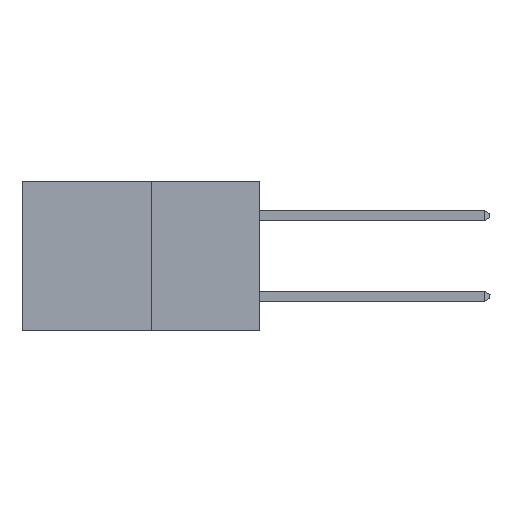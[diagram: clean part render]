
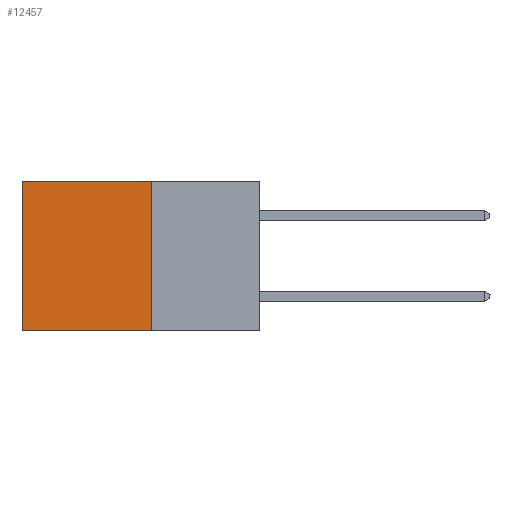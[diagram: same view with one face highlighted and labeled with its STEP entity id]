
A CAD part, left-side view. The second image highlights one B-rep face of the part: STEP entity #12457.
In plain terms, the highlighted planar face has unit normal (-1, 0, 0).
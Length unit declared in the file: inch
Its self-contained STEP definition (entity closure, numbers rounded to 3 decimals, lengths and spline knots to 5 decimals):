
#327 = VERTEX_POINT ( 'NONE', #22577 ) ;
#409 = VERTEX_POINT ( 'NONE', #3282 ) ;
#565 = VERTEX_POINT ( 'NONE', #15094 ) ;
#686 = ORIENTED_EDGE ( 'NONE', *, *, #25477, .T. ) ;
#914 = CARTESIAN_POINT ( 'NONE',  ( 0.277, 0.59, -0.37 ) ) ;
#937 = FACE_OUTER_BOUND ( 'NONE', #2817, .T. ) ;
#1234 = DIRECTION ( 'NONE',  ( 0., 1., 0. ) ) ;
#1362 = LINE ( 'NONE', #26528, #12355 ) ;
#2286 = DIRECTION ( 'NONE',  ( 0., 0., -1. ) ) ;
#2817 = EDGE_LOOP ( 'NONE', ( #7984, #17784, #15500, #686 ) ) ;
#3172 = DIRECTION ( 'NONE',  ( 0., 0., -1. ) ) ;
#3282 = CARTESIAN_POINT ( 'NONE',  ( 0.277, 0.59, 0. ) ) ;
#7818 = CARTESIAN_POINT ( 'NONE',  ( 0.277, 0.27, -0.37 ) ) ;
#7984 = ORIENTED_EDGE ( 'NONE', *, *, #8942, .T. ) ;
#8942 = EDGE_CURVE ( 'NONE', #409, #565, #15230, .T. ) ;
#10881 = VERTEX_POINT ( 'NONE', #18780 ) ;
#11003 = PLANE ( 'NONE',  #18610 ) ;
#12355 = VECTOR ( 'NONE', #22347, 39.37008 ) ;
#12457 = ADVANCED_FACE ( 'NONE', ( #937 ), #11003, .F. ) ;
#15094 = CARTESIAN_POINT ( 'NONE',  ( 0.277, 0.59, -0.37 ) ) ;
#15230 = LINE ( 'NONE', #914, #25888 ) ;
#15355 = DIRECTION ( 'NONE',  ( 1., 0., 0. ) ) ;
#15500 = ORIENTED_EDGE ( 'NONE', *, *, #17547, .F. ) ;
#15741 = VECTOR ( 'NONE', #25037, 39.37008 ) ;
#17052 = EDGE_CURVE ( 'NONE', #10881, #565, #25071, .T. ) ;
#17415 = CARTESIAN_POINT ( 'NONE',  ( 0.277, 0.27, -0.37 ) ) ;
#17547 = EDGE_CURVE ( 'NONE', #327, #10881, #1362, .T. ) ;
#17784 = ORIENTED_EDGE ( 'NONE', *, *, #17052, .F. ) ;
#18610 = AXIS2_PLACEMENT_3D ( 'NONE', #17415, #15355, #2286 ) ;
#18780 = CARTESIAN_POINT ( 'NONE',  ( 0.277, 0.27, -0.37 ) ) ;
#19413 = VECTOR ( 'NONE', #1234, 39.37008 ) ;
#20725 = LINE ( 'NONE', #22914, #15741 ) ;
#22347 = DIRECTION ( 'NONE',  ( 0., 0., -1. ) ) ;
#22577 = CARTESIAN_POINT ( 'NONE',  ( 0.277, 0.27, 0. ) ) ;
#22914 = CARTESIAN_POINT ( 'NONE',  ( 0.277, 0.27, 0. ) ) ;
#25037 = DIRECTION ( 'NONE',  ( 0., 1., 0. ) ) ;
#25071 = LINE ( 'NONE', #7818, #19413 ) ;
#25477 = EDGE_CURVE ( 'NONE', #327, #409, #20725, .T. ) ;
#25888 = VECTOR ( 'NONE', #3172, 39.37008 ) ;
#26528 = CARTESIAN_POINT ( 'NONE',  ( 0.277, 0.27, -0.37 ) ) ;
